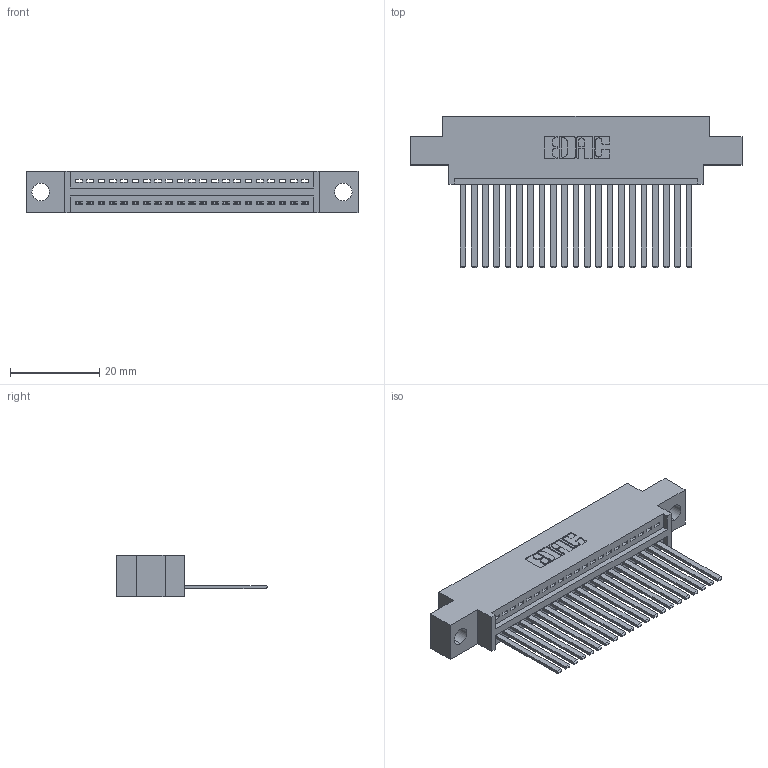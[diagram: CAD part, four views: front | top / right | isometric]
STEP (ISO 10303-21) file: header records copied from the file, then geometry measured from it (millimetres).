
FILE_DESCRIPTION (( 'STEP AP203' ), '1' );
FILE_NAME ('395-021-544-604.STEP', '2021-05-31T14:30:50', ( '' ), ( '' ), 'SwSTEP 2.0', 'SolidWorks 2020', '' );
FILE_SCHEMA (( 'CONFIG_CONTROL_DESIGN' ));
Length unit declared in the file: inch
Products named in the file (3): 345-292-001_345-293-144; 345 Part_0.170 Offset - 0.156 Dia-TI; 395-021-544-604
Assembly tree (22 placements, depth 2):
  395-021-544-604
    345 Part_0.170 Offset - 0.156 Dia-TI
    345-292-001_345-293-144  x21
Bounding box: 74.55 x 33.96 x 9.4 mm (x, y, z)
Volume: 6932.6 mm3; surface area: 9626.5 mm2
Topology: 22 solids, 22 shells, 1236 faces, 3707 edges, 2442 vertices
Faces by surface type: plane 854, cylinder 382
Entity records: 18999 total; most frequent: CARTESIAN_POINT 3301, ORIENTED_EDGE 3254, DIRECTION 2909, EDGE_CURVE 1627, VECTOR 1415, LINE 1415, VERTEX_POINT 1082, AXIS2_PLACEMENT_3D 747
